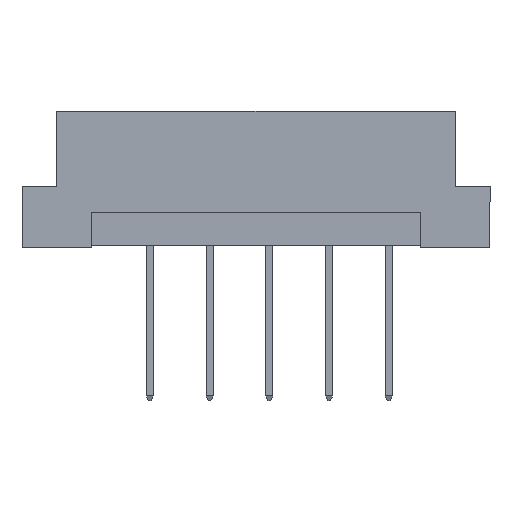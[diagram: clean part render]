
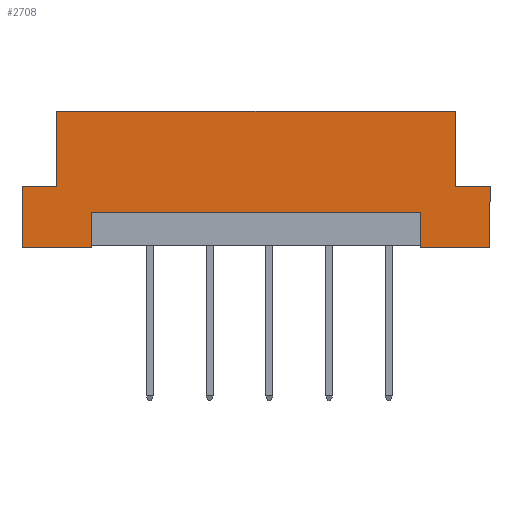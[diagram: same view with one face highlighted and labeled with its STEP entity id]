
A CAD part, front view. The second image highlights one B-rep face of the part: STEP entity #2708.
In plain terms, the highlighted planar face has unit normal (0, -1, 0).
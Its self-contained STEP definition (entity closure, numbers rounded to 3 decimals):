
#4 = VECTOR ( 'NONE', #800, 1000. ) ;
#99 = DIRECTION ( 'NONE',  ( 1., 0., 0. ) ) ;
#101 = EDGE_CURVE ( 'NONE', #4479, #4020, #1730, .T. ) ;
#111 = VECTOR ( 'NONE', #620, 1000. ) ;
#129 = EDGE_CURVE ( 'NONE', #673, #968, #2152, .T. ) ;
#281 = AXIS2_PLACEMENT_3D ( 'NONE', #3412, #747, #826 ) ;
#338 = VECTOR ( 'NONE', #980, 1000. ) ;
#357 = VECTOR ( 'NONE', #499, 1000. ) ;
#379 = ORIENTED_EDGE ( 'NONE', *, *, #3369, .F. ) ;
#481 = VECTOR ( 'NONE', #99, 1000. ) ;
#499 = DIRECTION ( 'NONE',  ( 0., 0., -1. ) ) ;
#505 = LINE ( 'NONE', #2453, #1217 ) ;
#555 = LINE ( 'NONE', #2556, #4753 ) ;
#620 = DIRECTION ( 'NONE',  ( 1., 0., 0. ) ) ;
#673 = VERTEX_POINT ( 'NONE', #3072 ) ;
#747 = DIRECTION ( 'NONE',  ( 0., 1., 0. ) ) ;
#800 = DIRECTION ( 'NONE',  ( 0., 0., 1. ) ) ;
#804 = DIRECTION ( 'NONE',  ( 0., 0., 1. ) ) ;
#826 = DIRECTION ( 'NONE',  ( -1., 0., 0. ) ) ;
#872 = CARTESIAN_POINT ( 'NONE',  ( -19.9, -4.3, 5.2 ) ) ;
#968 = VERTEX_POINT ( 'NONE', #1913 ) ;
#980 = DIRECTION ( 'NONE',  ( 0., 0., -1. ) ) ;
#997 = EDGE_CURVE ( 'NONE', #1655, #2166, #4718, .T. ) ;
#1005 = CARTESIAN_POINT ( 'NONE',  ( -14., -4.3, 3. ) ) ;
#1065 = CARTESIAN_POINT ( 'NONE',  ( -16.94, -4.3, 11.6 ) ) ;
#1074 = ORIENTED_EDGE ( 'NONE', *, *, #997, .F. ) ;
#1158 = CARTESIAN_POINT ( 'NONE',  ( 19.9, -4.3, 11.6 ) ) ;
#1217 = VECTOR ( 'NONE', #2817, 1000. ) ;
#1248 = EDGE_CURVE ( 'NONE', #3609, #2166, #2345, .T. ) ;
#1467 = CARTESIAN_POINT ( 'NONE',  ( 16.94, -4.3, 5.2 ) ) ;
#1566 = ORIENTED_EDGE ( 'NONE', *, *, #3382, .T. ) ;
#1567 = VERTEX_POINT ( 'NONE', #2989 ) ;
#1605 = LINE ( 'NONE', #2631, #4 ) ;
#1655 = VERTEX_POINT ( 'NONE', #1065 ) ;
#1730 = LINE ( 'NONE', #1005, #111 ) ;
#1913 = CARTESIAN_POINT ( 'NONE',  ( -14., -4.3, 0. ) ) ;
#2037 = VECTOR ( 'NONE', #4672, 1000. ) ;
#2055 = EDGE_CURVE ( 'NONE', #3609, #4263, #505, .T. ) ;
#2059 = CARTESIAN_POINT ( 'NONE',  ( 19.9, -4.3, 0. ) ) ;
#2108 = CARTESIAN_POINT ( 'NONE',  ( -14., -4.3, 0.2 ) ) ;
#2152 = LINE ( 'NONE', #3371, #3259 ) ;
#2166 = VERTEX_POINT ( 'NONE', #4976 ) ;
#2167 = CARTESIAN_POINT ( 'NONE',  ( 14., -4.3, 0. ) ) ;
#2274 = ORIENTED_EDGE ( 'NONE', *, *, #3972, .F. ) ;
#2345 = LINE ( 'NONE', #3071, #3373 ) ;
#2401 = LINE ( 'NONE', #872, #481 ) ;
#2453 = CARTESIAN_POINT ( 'NONE',  ( 19.9, -4.3, 5.2 ) ) ;
#2525 = VERTEX_POINT ( 'NONE', #2059 ) ;
#2556 = CARTESIAN_POINT ( 'NONE',  ( 19.9, -4.3, 0. ) ) ;
#2600 = VECTOR ( 'NONE', #804, 1000. ) ;
#2606 = VERTEX_POINT ( 'NONE', #2167 ) ;
#2631 = CARTESIAN_POINT ( 'NONE',  ( 14., -4.3, 0.2 ) ) ;
#2655 = EDGE_CURVE ( 'NONE', #2606, #2525, #555, .T. ) ;
#2708 = ADVANCED_FACE ( 'NONE', ( #4578 ), #3826, .F. ) ;
#2728 = CARTESIAN_POINT ( 'NONE',  ( 14., -4.3, 3. ) ) ;
#2806 = EDGE_CURVE ( 'NONE', #2606, #4020, #1605, .T. ) ;
#2817 = DIRECTION ( 'NONE',  ( 1., 0., 0. ) ) ;
#2825 = ORIENTED_EDGE ( 'NONE', *, *, #2055, .F. ) ;
#2925 = CARTESIAN_POINT ( 'NONE',  ( -16.94, -4.3, 5.2 ) ) ;
#2979 = CARTESIAN_POINT ( 'NONE',  ( -19.9, -4.3, 11.6 ) ) ;
#2989 = CARTESIAN_POINT ( 'NONE',  ( -16.94, -4.3, 5.2 ) ) ;
#3005 = LINE ( 'NONE', #2979, #338 ) ;
#3060 = ORIENTED_EDGE ( 'NONE', *, *, #129, .T. ) ;
#3071 = CARTESIAN_POINT ( 'NONE',  ( 16.94, -4.3, 5.2 ) ) ;
#3072 = CARTESIAN_POINT ( 'NONE',  ( -19.9, -4.3, 0. ) ) ;
#3222 = ORIENTED_EDGE ( 'NONE', *, *, #2655, .T. ) ;
#3259 = VECTOR ( 'NONE', #3295, 1000. ) ;
#3295 = DIRECTION ( 'NONE',  ( 1., 0., 0. ) ) ;
#3311 = LINE ( 'NONE', #2925, #2600 ) ;
#3369 = EDGE_CURVE ( 'NONE', #4263, #2525, #3811, .T. ) ;
#3371 = CARTESIAN_POINT ( 'NONE',  ( 19.9, -4.3, 0. ) ) ;
#3373 = VECTOR ( 'NONE', #4321, 1000. ) ;
#3382 = EDGE_CURVE ( 'NONE', #4154, #673, #3005, .T. ) ;
#3412 = CARTESIAN_POINT ( 'NONE',  ( 19.9, -4.3, 11.6 ) ) ;
#3567 = VECTOR ( 'NONE', #3708, 1000. ) ;
#3609 = VERTEX_POINT ( 'NONE', #1467 ) ;
#3708 = DIRECTION ( 'NONE',  ( 0., 0., -1. ) ) ;
#3748 = DIRECTION ( 'NONE',  ( 1., 0., 0. ) ) ;
#3811 = LINE ( 'NONE', #4977, #3567 ) ;
#3826 = PLANE ( 'NONE',  #281 ) ;
#3839 = ORIENTED_EDGE ( 'NONE', *, *, #1248, .T. ) ;
#3968 = ORIENTED_EDGE ( 'NONE', *, *, #5017, .F. ) ;
#3972 = EDGE_CURVE ( 'NONE', #1567, #1655, #3311, .T. ) ;
#4020 = VERTEX_POINT ( 'NONE', #2728 ) ;
#4103 = CARTESIAN_POINT ( 'NONE',  ( -19.9, -4.3, 5.2 ) ) ;
#4132 = LINE ( 'NONE', #2108, #357 ) ;
#4154 = VERTEX_POINT ( 'NONE', #4103 ) ;
#4155 = CARTESIAN_POINT ( 'NONE',  ( 19.9, -4.3, 5.2 ) ) ;
#4161 = ORIENTED_EDGE ( 'NONE', *, *, #4203, .F. ) ;
#4203 = EDGE_CURVE ( 'NONE', #4479, #968, #4132, .T. ) ;
#4263 = VERTEX_POINT ( 'NONE', #4155 ) ;
#4321 = DIRECTION ( 'NONE',  ( 0., 0., 1. ) ) ;
#4381 = EDGE_LOOP ( 'NONE', ( #4799, #5044, #3222, #379, #2825, #3839, #1074, #2274, #3968, #1566, #3060, #4161 ) ) ;
#4479 = VERTEX_POINT ( 'NONE', #4773 ) ;
#4578 = FACE_OUTER_BOUND ( 'NONE', #4381, .T. ) ;
#4672 = DIRECTION ( 'NONE',  ( 1., 0., 0. ) ) ;
#4718 = LINE ( 'NONE', #1158, #2037 ) ;
#4753 = VECTOR ( 'NONE', #3748, 1000. ) ;
#4773 = CARTESIAN_POINT ( 'NONE',  ( -14., -4.3, 3. ) ) ;
#4799 = ORIENTED_EDGE ( 'NONE', *, *, #101, .T. ) ;
#4976 = CARTESIAN_POINT ( 'NONE',  ( 16.94, -4.3, 11.6 ) ) ;
#4977 = CARTESIAN_POINT ( 'NONE',  ( 19.9, -4.3, 11.6 ) ) ;
#5017 = EDGE_CURVE ( 'NONE', #4154, #1567, #2401, .T. ) ;
#5044 = ORIENTED_EDGE ( 'NONE', *, *, #2806, .F. ) ;
